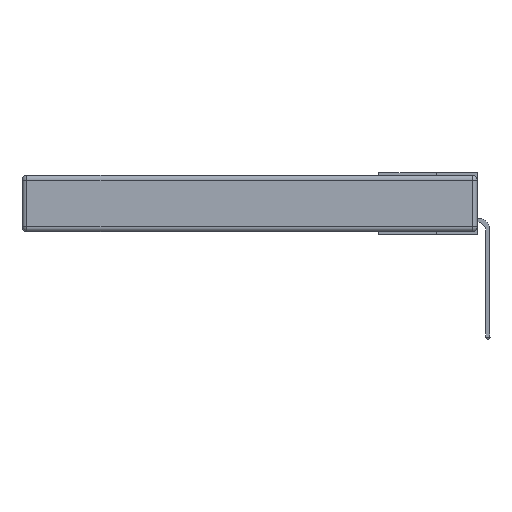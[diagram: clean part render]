
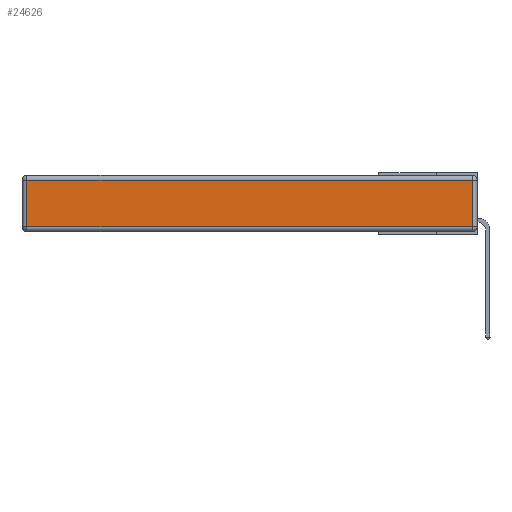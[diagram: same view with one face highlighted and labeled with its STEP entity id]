
A CAD part, left-side view. The second image highlights one B-rep face of the part: STEP entity #24626.
In plain terms, the highlighted planar face has unit normal (-1, 0, 0).
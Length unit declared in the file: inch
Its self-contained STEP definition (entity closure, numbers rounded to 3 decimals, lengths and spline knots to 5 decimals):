
#378 = VECTOR ( 'NONE', #8184, 39.37008 ) ;
#2079 = VECTOR ( 'NONE', #20311, 39.37008 ) ;
#2721 = ORIENTED_EDGE ( 'NONE', *, *, #4038, .T. ) ;
#4038 = EDGE_CURVE ( 'NONE', #4658, #17955, #28217, .T. ) ;
#4658 = VERTEX_POINT ( 'NONE', #27494 ) ;
#5957 = LINE ( 'NONE', #26660, #20477 ) ;
#6687 = CARTESIAN_POINT ( 'NONE',  ( 0., 2.72, -0.343 ) ) ;
#8184 = DIRECTION ( 'NONE',  ( 0., -1., 0. ) ) ;
#9287 = DIRECTION ( 'NONE',  ( -1., 0., 0. ) ) ;
#10664 = CARTESIAN_POINT ( 'NONE',  ( 0., 2.72, -0.313 ) ) ;
#10742 = CARTESIAN_POINT ( 'NONE',  ( 0., 2.72, -0.03 ) ) ;
#10929 = EDGE_CURVE ( 'NONE', #22475, #4658, #26263, .T. ) ;
#11667 = VERTEX_POINT ( 'NONE', #10742 ) ;
#12075 = AXIS2_PLACEMENT_3D ( 'NONE', #20333, #9287, #14044 ) ;
#14044 = DIRECTION ( 'NONE',  ( 0., 0., 1. ) ) ;
#14724 = CARTESIAN_POINT ( 'NONE',  ( 0., 0.03, -0.343 ) ) ;
#14854 = EDGE_CURVE ( 'NONE', #17955, #11667, #5957, .T. ) ;
#15014 = DIRECTION ( 'NONE',  ( 0., 0., 1. ) ) ;
#17284 = LINE ( 'NONE', #6687, #2079 ) ;
#17393 = EDGE_LOOP ( 'NONE', ( #20962, #2721, #20217, #24297 ) ) ;
#17955 = VERTEX_POINT ( 'NONE', #25206 ) ;
#18096 = PLANE ( 'NONE',  #12075 ) ;
#18202 = FACE_OUTER_BOUND ( 'NONE', #17393, .T. ) ;
#20217 = ORIENTED_EDGE ( 'NONE', *, *, #14854, .T. ) ;
#20311 = DIRECTION ( 'NONE',  ( 0., 0., -1. ) ) ;
#20333 = CARTESIAN_POINT ( 'NONE',  ( 0., 0., -0.343 ) ) ;
#20477 = VECTOR ( 'NONE', #23298, 39.37008 ) ;
#20962 = ORIENTED_EDGE ( 'NONE', *, *, #10929, .T. ) ;
#21435 = CARTESIAN_POINT ( 'NONE',  ( 0., 0., -0.313 ) ) ;
#22354 = VECTOR ( 'NONE', #15014, 39.37008 ) ;
#22475 = VERTEX_POINT ( 'NONE', #10664 ) ;
#22553 = EDGE_CURVE ( 'NONE', #11667, #22475, #17284, .T. ) ;
#23298 = DIRECTION ( 'NONE',  ( 0., 1., 0. ) ) ;
#24297 = ORIENTED_EDGE ( 'NONE', *, *, #22553, .T. ) ;
#24626 = ADVANCED_FACE ( 'NONE', ( #18202 ), #18096, .T. ) ;
#25206 = CARTESIAN_POINT ( 'NONE',  ( 0., 0.03, -0.03 ) ) ;
#26263 = LINE ( 'NONE', #21435, #378 ) ;
#26660 = CARTESIAN_POINT ( 'NONE',  ( 0., 2.75, -0.03 ) ) ;
#27494 = CARTESIAN_POINT ( 'NONE',  ( 0., 0.03, -0.313 ) ) ;
#28217 = LINE ( 'NONE', #14724, #22354 ) ;
